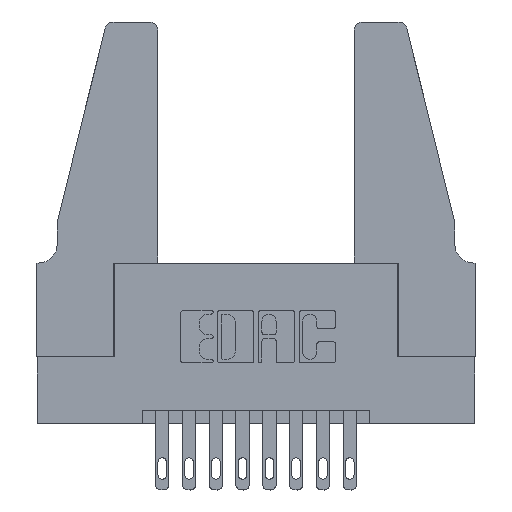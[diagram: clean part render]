
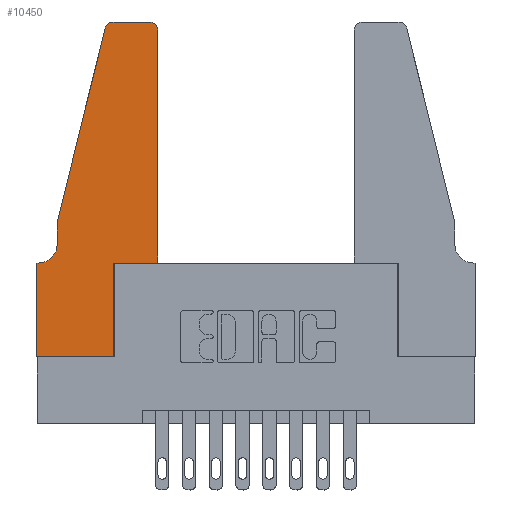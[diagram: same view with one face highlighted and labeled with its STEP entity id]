
A CAD part, top view. The second image highlights one B-rep face of the part: STEP entity #10450.
In plain terms, the highlighted planar face has unit normal (0, 0, 1).
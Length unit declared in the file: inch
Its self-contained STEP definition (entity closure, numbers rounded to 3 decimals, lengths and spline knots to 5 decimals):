
#39 = DIRECTION ( 'NONE',  ( 0., 0., 1. ) ) ;
#335 = VECTOR ( 'NONE', #8178, 39.37008 ) ;
#529 = VERTEX_POINT ( 'NONE', #10624 ) ;
#542 = CARTESIAN_POINT ( 'NONE',  ( 0.2865, 0., 0.37 ) ) ;
#738 = VECTOR ( 'NONE', #3278, 39.37008 ) ;
#905 = EDGE_CURVE ( 'NONE', #4280, #11310, #8139, .T. ) ;
#1075 = LINE ( 'NONE', #2002, #3123 ) ;
#1235 = CARTESIAN_POINT ( 'NONE',  ( 0.0755, 0.5, 0.37 ) ) ;
#1516 = CARTESIAN_POINT ( 'NONE',  ( 0.0755, 0.42, 0.37 ) ) ;
#1531 = CARTESIAN_POINT ( 'NONE',  ( 0., 0.35, 0.37 ) ) ;
#1659 = VERTEX_POINT ( 'NONE', #1516 ) ;
#2002 = CARTESIAN_POINT ( 'NONE',  ( 0.2605, 1.25, 0.37 ) ) ;
#2123 = DIRECTION ( 'NONE',  ( -1., 0., 0. ) ) ;
#2520 = CARTESIAN_POINT ( 'NONE',  ( 0.4505, 1.22, 0.37 ) ) ;
#2642 = VECTOR ( 'NONE', #3314, 39.37008 ) ;
#2779 = DIRECTION ( 'NONE',  ( 0., 0., 1. ) ) ;
#2800 = CARTESIAN_POINT ( 'NONE',  ( 0.284, 1.22, 0.37 ) ) ;
#3050 = CARTESIAN_POINT ( 'NONE',  ( 0.4205, 1.22, 0.37 ) ) ;
#3053 = ORIENTED_EDGE ( 'NONE', *, *, #11885, .T. ) ;
#3073 = EDGE_LOOP ( 'NONE', ( #11208, #5751, #7696, #11570, #10107, #8952, #6383, #3710, #3053, #3245, #10457, #5772 ) ) ;
#3088 = DIRECTION ( 'NONE',  ( 1., 0., 0. ) ) ;
#3106 = CIRCLE ( 'NONE', #7660, 0.03 ) ;
#3123 = VECTOR ( 'NONE', #2123, 39.37008 ) ;
#3237 = VECTOR ( 'NONE', #3088, 39.37008 ) ;
#3245 = ORIENTED_EDGE ( 'NONE', *, *, #12316, .T. ) ;
#3278 = DIRECTION ( 'NONE',  ( 0., -1., 0. ) ) ;
#3314 = DIRECTION ( 'NONE',  ( 0., 1., 0. ) ) ;
#3315 = EDGE_CURVE ( 'NONE', #9222, #4966, #10489, .T. ) ;
#3581 = AXIS2_PLACEMENT_3D ( 'NONE', #3050, #39, #5037 ) ;
#3583 = CARTESIAN_POINT ( 'NONE',  ( 0.4205, 1.25, 0.37 ) ) ;
#3645 = CARTESIAN_POINT ( 'NONE',  ( 0., 0., 0.37 ) ) ;
#3710 = ORIENTED_EDGE ( 'NONE', *, *, #7740, .T. ) ;
#4280 = VERTEX_POINT ( 'NONE', #9417 ) ;
#4377 = VERTEX_POINT ( 'NONE', #3645 ) ;
#4831 = LINE ( 'NONE', #8513, #7298 ) ;
#4890 = CARTESIAN_POINT ( 'NONE',  ( 0.0755, 0.35, 0.37 ) ) ;
#4933 = LINE ( 'NONE', #8147, #2642 ) ;
#4937 = CARTESIAN_POINT ( 'NONE',  ( 0.0055, 0.42, 0.37 ) ) ;
#4960 = VERTEX_POINT ( 'NONE', #3583 ) ;
#4966 = VERTEX_POINT ( 'NONE', #2520 ) ;
#5037 = DIRECTION ( 'NONE',  ( 1., 0., 0. ) ) ;
#5067 = EDGE_CURVE ( 'NONE', #11040, #4377, #4831, .T. ) ;
#5372 = LINE ( 'NONE', #12905, #3237 ) ;
#5467 = LINE ( 'NONE', #5479, #7831 ) ;
#5474 = VECTOR ( 'NONE', #11203, 39.37008 ) ;
#5479 = CARTESIAN_POINT ( 'NONE',  ( 0., 0., 0.37 ) ) ;
#5568 = VERTEX_POINT ( 'NONE', #10925 ) ;
#5751 = ORIENTED_EDGE ( 'NONE', *, *, #11727, .T. ) ;
#5772 = ORIENTED_EDGE ( 'NONE', *, *, #9831, .T. ) ;
#5894 = FACE_OUTER_BOUND ( 'NONE', #3073, .T. ) ;
#5918 = VERTEX_POINT ( 'NONE', #542 ) ;
#6012 = CARTESIAN_POINT ( 'NONE',  ( 0.0755, 0.5, 0.37 ) ) ;
#6383 = ORIENTED_EDGE ( 'NONE', *, *, #5067, .T. ) ;
#6566 = DIRECTION ( 'NONE',  ( 1., 0., 0. ) ) ;
#6758 = DIRECTION ( 'NONE',  ( 1., 0., 0. ) ) ;
#6869 = DIRECTION ( 'NONE',  ( 1., 0., 0. ) ) ;
#7298 = VECTOR ( 'NONE', #9386, 39.37008 ) ;
#7468 = CIRCLE ( 'NONE', #3581, 0.03 ) ;
#7660 = AXIS2_PLACEMENT_3D ( 'NONE', #2800, #9730, #6758 ) ;
#7675 = LINE ( 'NONE', #4890, #335 ) ;
#7696 = ORIENTED_EDGE ( 'NONE', *, *, #905, .T. ) ;
#7740 = EDGE_CURVE ( 'NONE', #4377, #5918, #5467, .T. ) ;
#7831 = VECTOR ( 'NONE', #6566, 39.37008 ) ;
#7836 = VECTOR ( 'NONE', #9860, 39.37008 ) ;
#7891 = EDGE_CURVE ( 'NONE', #10192, #11040, #7675, .T. ) ;
#7988 = AXIS2_PLACEMENT_3D ( 'NONE', #10848, #2779, #6869 ) ;
#8139 = LINE ( 'NONE', #6012, #5474 ) ;
#8147 = CARTESIAN_POINT ( 'NONE',  ( 0.2865, 0.35, 0.37 ) ) ;
#8178 = DIRECTION ( 'NONE',  ( -1., 0., 0. ) ) ;
#8412 = CARTESIAN_POINT ( 'NONE',  ( 0.0055, 0.35, 0.37 ) ) ;
#8513 = CARTESIAN_POINT ( 'NONE',  ( 0., 0., 0.37 ) ) ;
#8727 = CARTESIAN_POINT ( 'NONE',  ( 0.4505, 0.35, 0.37 ) ) ;
#8952 = ORIENTED_EDGE ( 'NONE', *, *, #7891, .T. ) ;
#8968 = DIRECTION ( 'NONE',  ( 0., 0., -1. ) ) ;
#9222 = VERTEX_POINT ( 'NONE', #8727 ) ;
#9386 = DIRECTION ( 'NONE',  ( 0., -1., 0. ) ) ;
#9417 = CARTESIAN_POINT ( 'NONE',  ( 0.25487, 1.22718, 0.37 ) ) ;
#9610 = CIRCLE ( 'NONE', #11281, 0.07 ) ;
#9730 = DIRECTION ( 'NONE',  ( 0., 0., 1. ) ) ;
#9749 = PLANE ( 'NONE',  #7988 ) ;
#9831 = EDGE_CURVE ( 'NONE', #4966, #4960, #7468, .T. ) ;
#9860 = DIRECTION ( 'NONE',  ( 0., 1., 0. ) ) ;
#9996 = DIRECTION ( 'NONE',  ( -1., 0., 0. ) ) ;
#10107 = ORIENTED_EDGE ( 'NONE', *, *, #11772, .T. ) ;
#10192 = VERTEX_POINT ( 'NONE', #8412 ) ;
#10255 = LINE ( 'NONE', #12963, #738 ) ;
#10450 = ADVANCED_FACE ( 'NONE', ( #5894 ), #9749, .T. ) ;
#10457 = ORIENTED_EDGE ( 'NONE', *, *, #3315, .T. ) ;
#10489 = LINE ( 'NONE', #10906, #7836 ) ;
#10624 = CARTESIAN_POINT ( 'NONE',  ( 0.2865, 0.35, 0.37 ) ) ;
#10848 = CARTESIAN_POINT ( 'NONE',  ( 0., 0.35, 0.37 ) ) ;
#10906 = CARTESIAN_POINT ( 'NONE',  ( 0.4505, 0.35, 0.37 ) ) ;
#10925 = CARTESIAN_POINT ( 'NONE',  ( 0.284, 1.25, 0.37 ) ) ;
#11040 = VERTEX_POINT ( 'NONE', #1531 ) ;
#11193 = EDGE_CURVE ( 'NONE', #4960, #5568, #1075, .T. ) ;
#11203 = DIRECTION ( 'NONE',  ( -0.239, -0.971, 0. ) ) ;
#11208 = ORIENTED_EDGE ( 'NONE', *, *, #11193, .T. ) ;
#11281 = AXIS2_PLACEMENT_3D ( 'NONE', #4937, #8968, #9996 ) ;
#11310 = VERTEX_POINT ( 'NONE', #1235 ) ;
#11570 = ORIENTED_EDGE ( 'NONE', *, *, #11666, .T. ) ;
#11666 = EDGE_CURVE ( 'NONE', #11310, #1659, #10255, .T. ) ;
#11727 = EDGE_CURVE ( 'NONE', #5568, #4280, #3106, .T. ) ;
#11772 = EDGE_CURVE ( 'NONE', #1659, #10192, #9610, .T. ) ;
#11885 = EDGE_CURVE ( 'NONE', #5918, #529, #4933, .T. ) ;
#12316 = EDGE_CURVE ( 'NONE', #529, #9222, #5372, .T. ) ;
#12905 = CARTESIAN_POINT ( 'NONE',  ( 0.4505, 0.35, 0.37 ) ) ;
#12963 = CARTESIAN_POINT ( 'NONE',  ( 0.0755, 0.5, 0.37 ) ) ;
